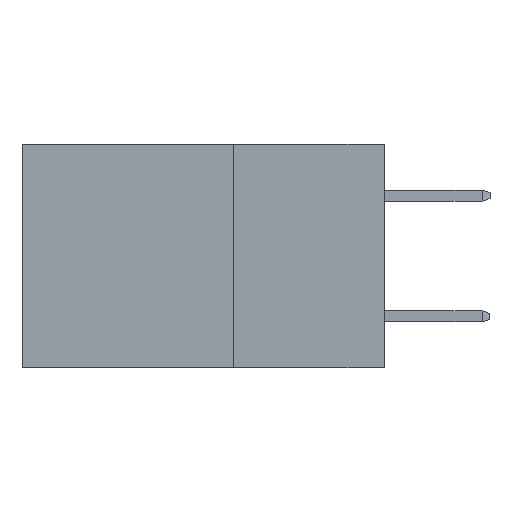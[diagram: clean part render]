
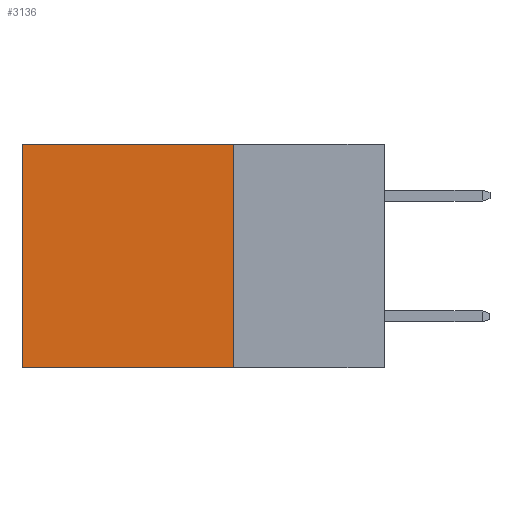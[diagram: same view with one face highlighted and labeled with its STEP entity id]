
A CAD part, left-side view. The second image highlights one B-rep face of the part: STEP entity #3136.
In plain terms, the highlighted planar face has unit normal (-1, 0, 0).
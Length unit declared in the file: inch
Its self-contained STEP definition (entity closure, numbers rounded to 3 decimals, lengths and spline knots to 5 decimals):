
#636 = LINE ( 'NONE', #8661, #2735 ) ;
#937 = LINE ( 'NONE', #9781, #7911 ) ;
#1120 = AXIS2_PLACEMENT_3D ( 'NONE', #7993, #10536, #5431 ) ;
#1511 = EDGE_CURVE ( 'NONE', #4620, #5262, #9071, .T. ) ;
#1565 = DIRECTION ( 'NONE',  ( 0., 0., -1. ) ) ;
#1880 = CARTESIAN_POINT ( 'NONE',  ( 0.298, 0.6, 0. ) ) ;
#2317 = ORIENTED_EDGE ( 'NONE', *, *, #1511, .F. ) ;
#2375 = FACE_OUTER_BOUND ( 'NONE', #11103, .T. ) ;
#2735 = VECTOR ( 'NONE', #4384, 39.37008 ) ;
#2804 = ORIENTED_EDGE ( 'NONE', *, *, #6582, .T. ) ;
#3136 = ADVANCED_FACE ( 'NONE', ( #2375 ), #7144, .F. ) ;
#3354 = ORIENTED_EDGE ( 'NONE', *, *, #6103, .F. ) ;
#4384 = DIRECTION ( 'NONE',  ( 0., 0., -1. ) ) ;
#4477 = LINE ( 'NONE', #8395, #6484 ) ;
#4593 = CARTESIAN_POINT ( 'NONE',  ( 0.298, 0.25, 0. ) ) ;
#4620 = VERTEX_POINT ( 'NONE', #4828 ) ;
#4828 = CARTESIAN_POINT ( 'NONE',  ( 0.298, 0.25, 0. ) ) ;
#5262 = VERTEX_POINT ( 'NONE', #9162 ) ;
#5431 = DIRECTION ( 'NONE',  ( 0., 0., -1. ) ) ;
#5456 = VERTEX_POINT ( 'NONE', #7655 ) ;
#5498 = DIRECTION ( 'NONE',  ( 0., 1., 0. ) ) ;
#6103 = EDGE_CURVE ( 'NONE', #5262, #5456, #937, .T. ) ;
#6245 = ORIENTED_EDGE ( 'NONE', *, *, #10057, .T. ) ;
#6484 = VECTOR ( 'NONE', #9230, 39.37008 ) ;
#6582 = EDGE_CURVE ( 'NONE', #8096, #5456, #636, .T. ) ;
#7144 = PLANE ( 'NONE',  #1120 ) ;
#7655 = CARTESIAN_POINT ( 'NONE',  ( 0.298, 0.6, -0.37 ) ) ;
#7911 = VECTOR ( 'NONE', #5498, 39.37008 ) ;
#7993 = CARTESIAN_POINT ( 'NONE',  ( 0.298, 0.25, 0. ) ) ;
#8096 = VERTEX_POINT ( 'NONE', #1880 ) ;
#8395 = CARTESIAN_POINT ( 'NONE',  ( 0.298, 0.25, 0. ) ) ;
#8661 = CARTESIAN_POINT ( 'NONE',  ( 0.298, 0.6, 0. ) ) ;
#9071 = LINE ( 'NONE', #4593, #10758 ) ;
#9162 = CARTESIAN_POINT ( 'NONE',  ( 0.298, 0.25, -0.37 ) ) ;
#9230 = DIRECTION ( 'NONE',  ( 0., 1., 0. ) ) ;
#9781 = CARTESIAN_POINT ( 'NONE',  ( 0.298, 0.25, -0.37 ) ) ;
#10057 = EDGE_CURVE ( 'NONE', #4620, #8096, #4477, .T. ) ;
#10536 = DIRECTION ( 'NONE',  ( 1., 0., 0. ) ) ;
#10758 = VECTOR ( 'NONE', #1565, 39.37008 ) ;
#11103 = EDGE_LOOP ( 'NONE', ( #2804, #3354, #2317, #6245 ) ) ;
